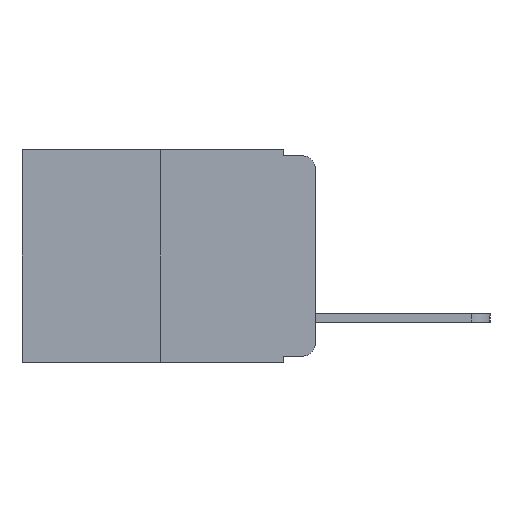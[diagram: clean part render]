
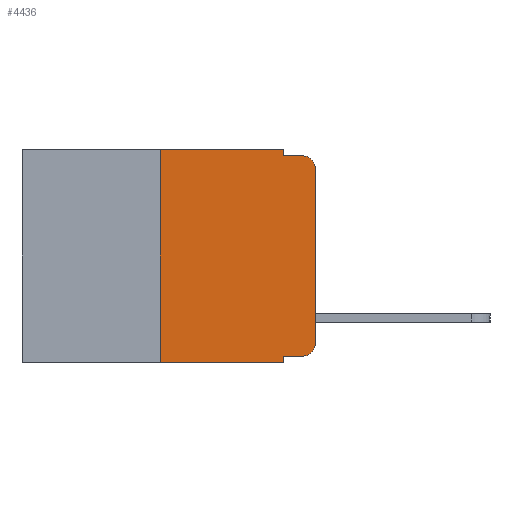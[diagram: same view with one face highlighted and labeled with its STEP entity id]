
A CAD part, left-side view. The second image highlights one B-rep face of the part: STEP entity #4436.
In plain terms, the highlighted planar face has unit normal (-1, 0, 0).
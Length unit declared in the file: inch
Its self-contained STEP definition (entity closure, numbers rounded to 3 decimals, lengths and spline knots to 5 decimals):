
#136 = CARTESIAN_POINT ( 'NONE',  ( 0., 0.051, -0.333 ) ) ;
#317 = VECTOR ( 'NONE', #11199, 39.37008 ) ;
#512 = ORIENTED_EDGE ( 'NONE', *, *, #10653, .F. ) ;
#819 = VERTEX_POINT ( 'NONE', #15116 ) ;
#980 = CARTESIAN_POINT ( 'NONE',  ( 0., 0.051, 0. ) ) ;
#1271 = DIRECTION ( 'NONE',  ( 0., 0., -1. ) ) ;
#1283 = VERTEX_POINT ( 'NONE', #2498 ) ;
#2208 = VERTEX_POINT ( 'NONE', #6822 ) ;
#2267 = ORIENTED_EDGE ( 'NONE', *, *, #12899, .F. ) ;
#2498 = CARTESIAN_POINT ( 'NONE',  ( 0., 0., -0.03 ) ) ;
#2556 = ORIENTED_EDGE ( 'NONE', *, *, #12991, .T. ) ;
#3194 = VERTEX_POINT ( 'NONE', #9022 ) ;
#3198 = ORIENTED_EDGE ( 'NONE', *, *, #8151, .T. ) ;
#3207 = CARTESIAN_POINT ( 'NONE',  ( 0., 0.25, 0. ) ) ;
#3827 = EDGE_CURVE ( 'NONE', #819, #11625, #7680, .T. ) ;
#3930 = ORIENTED_EDGE ( 'NONE', *, *, #12231, .T. ) ;
#3982 = CIRCLE ( 'NONE', #12195, 0.02 ) ;
#4277 = ORIENTED_EDGE ( 'NONE', *, *, #3827, .F. ) ;
#4390 = VECTOR ( 'NONE', #4658, 39.37008 ) ;
#4436 = ADVANCED_FACE ( 'NONE', ( #12813 ), #10819, .F. ) ;
#4658 = DIRECTION ( 'NONE',  ( 0., -1., 0. ) ) ;
#4780 = ORIENTED_EDGE ( 'NONE', *, *, #13735, .F. ) ;
#4837 = CARTESIAN_POINT ( 'NONE',  ( 0., 0.02, -0.313 ) ) ;
#4887 = ORIENTED_EDGE ( 'NONE', *, *, #14478, .F. ) ;
#4901 = ORIENTED_EDGE ( 'NONE', *, *, #9541, .T. ) ;
#5083 = ORIENTED_EDGE ( 'NONE', *, *, #13181, .T. ) ;
#5097 = CARTESIAN_POINT ( 'NONE',  ( 0., 0., 0. ) ) ;
#5118 = AXIS2_PLACEMENT_3D ( 'NONE', #6031, #14178, #7206 ) ;
#5214 = CARTESIAN_POINT ( 'NONE',  ( 0., 0.473, -0.343 ) ) ;
#5362 = VECTOR ( 'NONE', #1271, 39.37008 ) ;
#5651 = LINE ( 'NONE', #5214, #11967 ) ;
#6031 = CARTESIAN_POINT ( 'NONE',  ( 0., 0.02, -0.03 ) ) ;
#6147 = DIRECTION ( 'NONE',  ( 0., 0., -1. ) ) ;
#6322 = CARTESIAN_POINT ( 'NONE',  ( 0., 0.02, -0.01 ) ) ;
#6729 = LINE ( 'NONE', #5097, #317 ) ;
#6779 = CARTESIAN_POINT ( 'NONE',  ( 0., 0.051, 0. ) ) ;
#6822 = CARTESIAN_POINT ( 'NONE',  ( 0., 0.25, -0.343 ) ) ;
#6997 = VERTEX_POINT ( 'NONE', #980 ) ;
#7005 = CARTESIAN_POINT ( 'NONE',  ( 0., 0.051, -0.01 ) ) ;
#7124 = DIRECTION ( 'NONE',  ( 0., -1., 0. ) ) ;
#7206 = DIRECTION ( 'NONE',  ( 0., 0., -1. ) ) ;
#7347 = VERTEX_POINT ( 'NONE', #136 ) ;
#7680 = LINE ( 'NONE', #7005, #4390 ) ;
#7711 = CARTESIAN_POINT ( 'NONE',  ( 0., 0.051, 0. ) ) ;
#7733 = AXIS2_PLACEMENT_3D ( 'NONE', #8750, #15844, #12617 ) ;
#8151 = EDGE_CURVE ( 'NONE', #1283, #11625, #11831, .T. ) ;
#8535 = LINE ( 'NONE', #7711, #5362 ) ;
#8750 = CARTESIAN_POINT ( 'NONE',  ( 0., 0.473, 0. ) ) ;
#8823 = CARTESIAN_POINT ( 'NONE',  ( 0., 0.25, 0. ) ) ;
#9022 = CARTESIAN_POINT ( 'NONE',  ( 0., 0.02, -0.333 ) ) ;
#9510 = CARTESIAN_POINT ( 'NONE',  ( 0., 0., -0.313 ) ) ;
#9541 = EDGE_CURVE ( 'NONE', #2208, #12918, #5651, .T. ) ;
#9575 = DIRECTION ( 'NONE',  ( 0., -1., 0. ) ) ;
#9621 = CARTESIAN_POINT ( 'NONE',  ( 0., 0.051, -0.333 ) ) ;
#10596 = VECTOR ( 'NONE', #15718, 39.37008 ) ;
#10653 = EDGE_CURVE ( 'NONE', #6997, #819, #15618, .T. ) ;
#10753 = VERTEX_POINT ( 'NONE', #3207 ) ;
#10819 = PLANE ( 'NONE',  #7733 ) ;
#11018 = EDGE_LOOP ( 'NONE', ( #5083, #3198, #4277, #512, #2267, #4887, #4901, #4780, #2556, #3930 ) ) ;
#11199 = DIRECTION ( 'NONE',  ( 0., 0., 1. ) ) ;
#11362 = LINE ( 'NONE', #9621, #14354 ) ;
#11462 = VERTEX_POINT ( 'NONE', #9510 ) ;
#11625 = VERTEX_POINT ( 'NONE', #6322 ) ;
#11831 = CIRCLE ( 'NONE', #5118, 0.02 ) ;
#11967 = VECTOR ( 'NONE', #12374, 39.37008 ) ;
#12195 = AXIS2_PLACEMENT_3D ( 'NONE', #4837, #13183, #6147 ) ;
#12231 = EDGE_CURVE ( 'NONE', #3194, #11462, #3982, .T. ) ;
#12301 = VECTOR ( 'NONE', #13754, 39.37008 ) ;
#12374 = DIRECTION ( 'NONE',  ( 0., -1., 0. ) ) ;
#12617 = DIRECTION ( 'NONE',  ( 0., 0., -1. ) ) ;
#12788 = LINE ( 'NONE', #14089, #15402 ) ;
#12813 = FACE_OUTER_BOUND ( 'NONE', #11018, .T. ) ;
#12899 = EDGE_CURVE ( 'NONE', #10753, #6997, #12788, .T. ) ;
#12918 = VERTEX_POINT ( 'NONE', #13032 ) ;
#12962 = LINE ( 'NONE', #8823, #10596 ) ;
#12991 = EDGE_CURVE ( 'NONE', #7347, #3194, #11362, .T. ) ;
#13032 = CARTESIAN_POINT ( 'NONE',  ( 0., 0.051, -0.343 ) ) ;
#13181 = EDGE_CURVE ( 'NONE', #11462, #1283, #6729, .T. ) ;
#13183 = DIRECTION ( 'NONE',  ( -1., 0., 0. ) ) ;
#13735 = EDGE_CURVE ( 'NONE', #7347, #12918, #8535, .T. ) ;
#13754 = DIRECTION ( 'NONE',  ( 0., 0., -1. ) ) ;
#14089 = CARTESIAN_POINT ( 'NONE',  ( 0., 0.473, 0. ) ) ;
#14178 = DIRECTION ( 'NONE',  ( -1., 0., 0. ) ) ;
#14354 = VECTOR ( 'NONE', #9575, 39.37008 ) ;
#14478 = EDGE_CURVE ( 'NONE', #2208, #10753, #12962, .T. ) ;
#15116 = CARTESIAN_POINT ( 'NONE',  ( 0., 0.051, -0.01 ) ) ;
#15402 = VECTOR ( 'NONE', #7124, 39.37008 ) ;
#15618 = LINE ( 'NONE', #6779, #12301 ) ;
#15718 = DIRECTION ( 'NONE',  ( 0., 0., 1. ) ) ;
#15844 = DIRECTION ( 'NONE',  ( 1., 0., 0. ) ) ;
